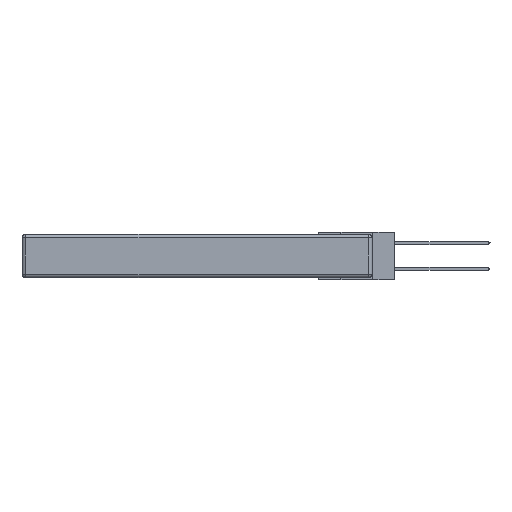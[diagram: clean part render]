
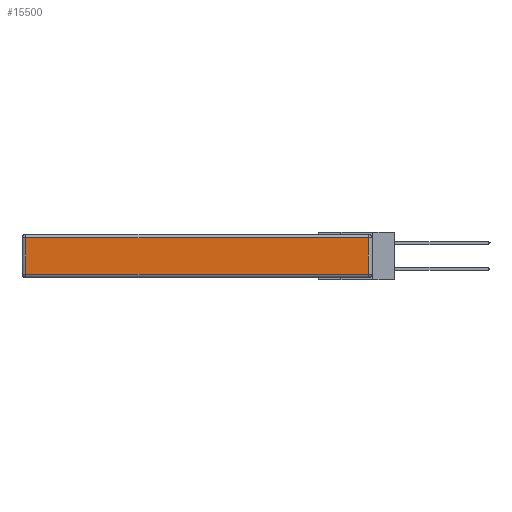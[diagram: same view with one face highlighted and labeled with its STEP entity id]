
A CAD part, left-side view. The second image highlights one B-rep face of the part: STEP entity #15500.
In plain terms, the highlighted planar face has unit normal (-1, 0, 0).
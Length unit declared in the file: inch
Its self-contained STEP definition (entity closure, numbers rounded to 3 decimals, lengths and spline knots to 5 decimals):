
#1207 = EDGE_CURVE ( 'NONE', #23105, #20128, #14169, .T. ) ;
#1545 = LINE ( 'NONE', #16213, #13203 ) ;
#1843 = VECTOR ( 'NONE', #21568, 39.37008 ) ;
#2560 = VECTOR ( 'NONE', #16534, 39.37008 ) ;
#3723 = EDGE_CURVE ( 'NONE', #20128, #7381, #17206, .T. ) ;
#4489 = VECTOR ( 'NONE', #4787, 39.37008 ) ;
#4787 = DIRECTION ( 'NONE',  ( 0., 0., 1. ) ) ;
#5254 = DIRECTION ( 'NONE',  ( 0., 0., -1. ) ) ;
#5610 = CARTESIAN_POINT ( 'NONE',  ( 0., 0.03, -0.03 ) ) ;
#5953 = CARTESIAN_POINT ( 'NONE',  ( 0., 2.72, -0.03 ) ) ;
#6483 = AXIS2_PLACEMENT_3D ( 'NONE', #17796, #19979, #6837 ) ;
#6835 = EDGE_CURVE ( 'NONE', #7381, #26911, #28281, .T. ) ;
#6837 = DIRECTION ( 'NONE',  ( 0., 0., 1. ) ) ;
#7381 = VERTEX_POINT ( 'NONE', #5610 ) ;
#8699 = CARTESIAN_POINT ( 'NONE',  ( 0., 0., -0.313 ) ) ;
#9786 = CARTESIAN_POINT ( 'NONE',  ( 0., 2.72, -0.313 ) ) ;
#9810 = CARTESIAN_POINT ( 'NONE',  ( 0., 2.75, -0.03 ) ) ;
#10507 = FACE_OUTER_BOUND ( 'NONE', #21745, .T. ) ;
#12970 = ORIENTED_EDGE ( 'NONE', *, *, #3723, .T. ) ;
#13203 = VECTOR ( 'NONE', #5254, 39.37008 ) ;
#14169 = LINE ( 'NONE', #8699, #1843 ) ;
#15026 = ORIENTED_EDGE ( 'NONE', *, *, #16502, .T. ) ;
#15500 = ADVANCED_FACE ( 'NONE', ( #10507 ), #22429, .T. ) ;
#15721 = CARTESIAN_POINT ( 'NONE',  ( 0., 0.03, -0.343 ) ) ;
#16213 = CARTESIAN_POINT ( 'NONE',  ( 0., 2.72, -0.343 ) ) ;
#16502 = EDGE_CURVE ( 'NONE', #26911, #23105, #1545, .T. ) ;
#16534 = DIRECTION ( 'NONE',  ( 0., 1., 0. ) ) ;
#17206 = LINE ( 'NONE', #15721, #4489 ) ;
#17796 = CARTESIAN_POINT ( 'NONE',  ( 0., 0., -0.343 ) ) ;
#17883 = ORIENTED_EDGE ( 'NONE', *, *, #1207, .T. ) ;
#18662 = CARTESIAN_POINT ( 'NONE',  ( 0., 0.03, -0.313 ) ) ;
#19054 = ORIENTED_EDGE ( 'NONE', *, *, #6835, .T. ) ;
#19979 = DIRECTION ( 'NONE',  ( -1., 0., 0. ) ) ;
#20128 = VERTEX_POINT ( 'NONE', #18662 ) ;
#21568 = DIRECTION ( 'NONE',  ( 0., -1., 0. ) ) ;
#21745 = EDGE_LOOP ( 'NONE', ( #17883, #12970, #19054, #15026 ) ) ;
#22429 = PLANE ( 'NONE',  #6483 ) ;
#23105 = VERTEX_POINT ( 'NONE', #9786 ) ;
#26911 = VERTEX_POINT ( 'NONE', #5953 ) ;
#28281 = LINE ( 'NONE', #9810, #2560 ) ;
